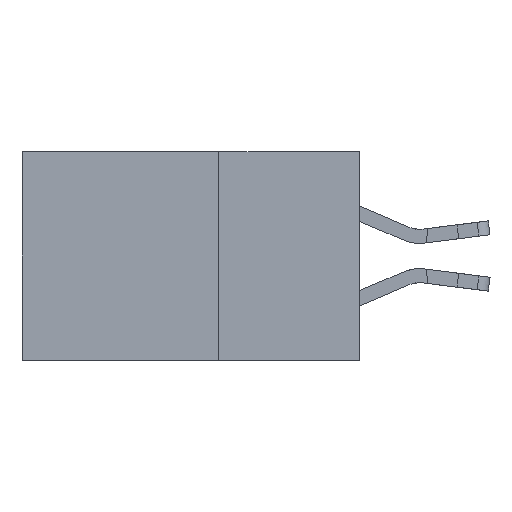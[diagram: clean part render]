
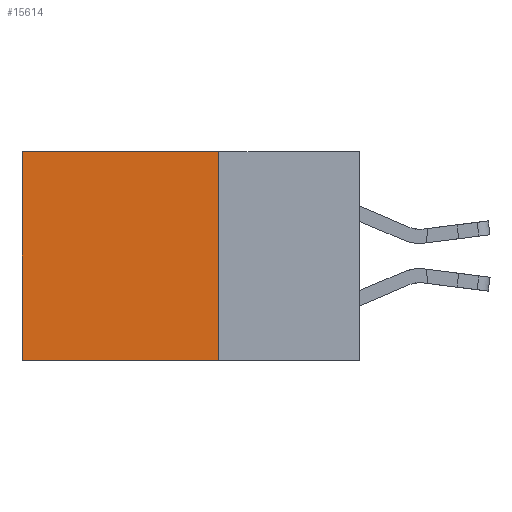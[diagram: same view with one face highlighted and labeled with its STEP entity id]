
A CAD part, left-side view. The second image highlights one B-rep face of the part: STEP entity #15614.
In plain terms, the highlighted planar face has unit normal (-1, 0, 0).
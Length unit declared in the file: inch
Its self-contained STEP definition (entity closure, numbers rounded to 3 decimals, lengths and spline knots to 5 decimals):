
#1491 = AXIS2_PLACEMENT_3D ( 'NONE', #12987, #1959, #25672 ) ;
#1931 = EDGE_CURVE ( 'NONE', #3075, #14438, #4589, .T. ) ;
#1959 = DIRECTION ( 'NONE',  ( 1., 0., 0. ) ) ;
#3075 = VERTEX_POINT ( 'NONE', #22224 ) ;
#3239 = ORIENTED_EDGE ( 'NONE', *, *, #1931, .F. ) ;
#4558 = LINE ( 'NONE', #21735, #10148 ) ;
#4589 = LINE ( 'NONE', #13189, #9193 ) ;
#5923 = FACE_OUTER_BOUND ( 'NONE', #12686, .T. ) ;
#7421 = EDGE_CURVE ( 'NONE', #14438, #14682, #17880, .T. ) ;
#7593 = CARTESIAN_POINT ( 'NONE',  ( 0.2875, 0.25, -0.37 ) ) ;
#9193 = VECTOR ( 'NONE', #21778, 39.37008 ) ;
#10148 = VECTOR ( 'NONE', #13557, 39.37008 ) ;
#10604 = PLANE ( 'NONE',  #1491 ) ;
#11877 = VECTOR ( 'NONE', #15633, 39.37008 ) ;
#11951 = ORIENTED_EDGE ( 'NONE', *, *, #26237, .T. ) ;
#12686 = EDGE_LOOP ( 'NONE', ( #11951, #17611, #3239, #16534 ) ) ;
#12987 = CARTESIAN_POINT ( 'NONE',  ( 0.2875, 0.25, 0. ) ) ;
#13155 = CARTESIAN_POINT ( 'NONE',  ( 0.2875, 0.6, 0. ) ) ;
#13189 = CARTESIAN_POINT ( 'NONE',  ( 0.2875, 0.25, 0. ) ) ;
#13557 = DIRECTION ( 'NONE',  ( 0., 0., -1. ) ) ;
#13667 = CARTESIAN_POINT ( 'NONE',  ( 0.2875, 0.25, -0.37 ) ) ;
#14263 = CARTESIAN_POINT ( 'NONE',  ( 0.2875, 0.25, 0. ) ) ;
#14438 = VERTEX_POINT ( 'NONE', #7593 ) ;
#14682 = VERTEX_POINT ( 'NONE', #23079 ) ;
#15282 = VERTEX_POINT ( 'NONE', #13155 ) ;
#15614 = ADVANCED_FACE ( 'NONE', ( #5923 ), #10604, .F. ) ;
#15633 = DIRECTION ( 'NONE',  ( 0., 1., 0. ) ) ;
#16534 = ORIENTED_EDGE ( 'NONE', *, *, #18920, .T. ) ;
#17611 = ORIENTED_EDGE ( 'NONE', *, *, #7421, .F. ) ;
#17880 = LINE ( 'NONE', #13667, #11877 ) ;
#18920 = EDGE_CURVE ( 'NONE', #3075, #15282, #22158, .T. ) ;
#21735 = CARTESIAN_POINT ( 'NONE',  ( 0.2875, 0.6, 0. ) ) ;
#21778 = DIRECTION ( 'NONE',  ( 0., 0., -1. ) ) ;
#22158 = LINE ( 'NONE', #14263, #27682 ) ;
#22224 = CARTESIAN_POINT ( 'NONE',  ( 0.2875, 0.25, 0. ) ) ;
#23079 = CARTESIAN_POINT ( 'NONE',  ( 0.2875, 0.6, -0.37 ) ) ;
#23126 = DIRECTION ( 'NONE',  ( 0., 1., 0. ) ) ;
#25672 = DIRECTION ( 'NONE',  ( 0., 0., -1. ) ) ;
#26237 = EDGE_CURVE ( 'NONE', #15282, #14682, #4558, .T. ) ;
#27682 = VECTOR ( 'NONE', #23126, 39.37008 ) ;
